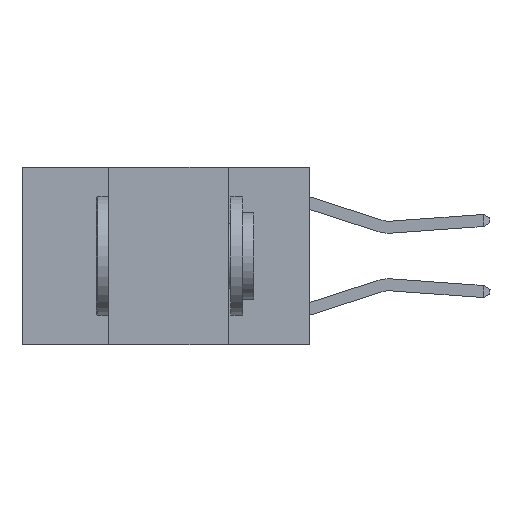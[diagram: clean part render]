
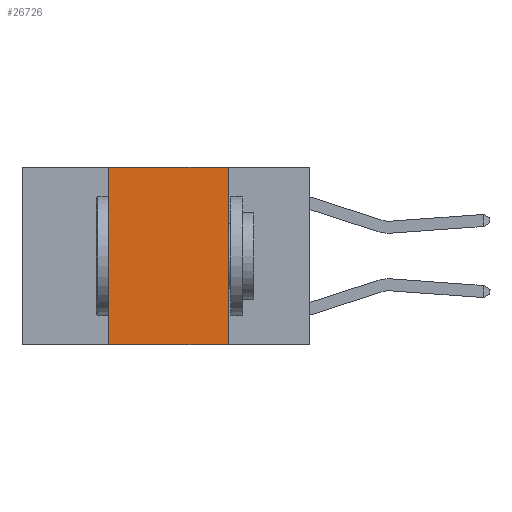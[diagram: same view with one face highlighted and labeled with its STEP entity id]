
A CAD part, left-side view. The second image highlights one B-rep face of the part: STEP entity #26726.
In plain terms, the highlighted planar face has unit normal (-1, 0, 0).
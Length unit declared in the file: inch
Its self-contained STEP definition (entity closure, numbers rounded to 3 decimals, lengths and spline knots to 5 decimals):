
#485 = CARTESIAN_POINT ( 'NONE',  ( 0., 0.17, -0.37 ) ) ;
#1969 = VERTEX_POINT ( 'NONE', #8982 ) ;
#2531 = EDGE_CURVE ( 'NONE', #25763, #14042, #25010, .T. ) ;
#5132 = LINE ( 'NONE', #27263, #9984 ) ;
#6787 = DIRECTION ( 'NONE',  ( 0., -1., 0. ) ) ;
#6900 = CARTESIAN_POINT ( 'NONE',  ( 0., 0.17, 0. ) ) ;
#8418 = EDGE_CURVE ( 'NONE', #1969, #25763, #23509, .T. ) ;
#8488 = ORIENTED_EDGE ( 'NONE', *, *, #8418, .F. ) ;
#8982 = CARTESIAN_POINT ( 'NONE',  ( 0., 0.42, 0. ) ) ;
#9158 = CARTESIAN_POINT ( 'NONE',  ( 0., 0.42, -0.37 ) ) ;
#9280 = PLANE ( 'NONE',  #16849 ) ;
#9984 = VECTOR ( 'NONE', #29518, 39.37008 ) ;
#11680 = DIRECTION ( 'NONE',  ( 0., 0., -1. ) ) ;
#13084 = VERTEX_POINT ( 'NONE', #9158 ) ;
#14012 = DIRECTION ( 'NONE',  ( 0., 0., -1. ) ) ;
#14042 = VERTEX_POINT ( 'NONE', #485 ) ;
#15091 = DIRECTION ( 'NONE',  ( 0., 0., 1. ) ) ;
#15138 = LINE ( 'NONE', #17421, #20608 ) ;
#15577 = ORIENTED_EDGE ( 'NONE', *, *, #16954, .F. ) ;
#16849 = AXIS2_PLACEMENT_3D ( 'NONE', #27868, #25731, #11680 ) ;
#16954 = EDGE_CURVE ( 'NONE', #13084, #1969, #15138, .T. ) ;
#17421 = CARTESIAN_POINT ( 'NONE',  ( 0., 0.42, 0. ) ) ;
#17814 = CARTESIAN_POINT ( 'NONE',  ( 0., 0.17, 0. ) ) ;
#20057 = FACE_OUTER_BOUND ( 'NONE', #29078, .T. ) ;
#20608 = VECTOR ( 'NONE', #15091, 39.37008 ) ;
#21649 = EDGE_CURVE ( 'NONE', #13084, #14042, #5132, .T. ) ;
#21776 = ORIENTED_EDGE ( 'NONE', *, *, #21649, .T. ) ;
#23304 = CARTESIAN_POINT ( 'NONE',  ( 0., 0.6, 0. ) ) ;
#23509 = LINE ( 'NONE', #23304, #24247 ) ;
#24247 = VECTOR ( 'NONE', #6787, 39.37008 ) ;
#25010 = LINE ( 'NONE', #6900, #25736 ) ;
#25731 = DIRECTION ( 'NONE',  ( 1., 0., 0. ) ) ;
#25736 = VECTOR ( 'NONE', #14012, 39.37008 ) ;
#25763 = VERTEX_POINT ( 'NONE', #17814 ) ;
#26468 = ORIENTED_EDGE ( 'NONE', *, *, #2531, .F. ) ;
#26726 = ADVANCED_FACE ( 'NONE', ( #20057 ), #9280, .F. ) ;
#27263 = CARTESIAN_POINT ( 'NONE',  ( 0., 0.6, -0.37 ) ) ;
#27868 = CARTESIAN_POINT ( 'NONE',  ( 0., 0.6, 0. ) ) ;
#29078 = EDGE_LOOP ( 'NONE', ( #26468, #8488, #15577, #21776 ) ) ;
#29518 = DIRECTION ( 'NONE',  ( 0., -1., 0. ) ) ;
